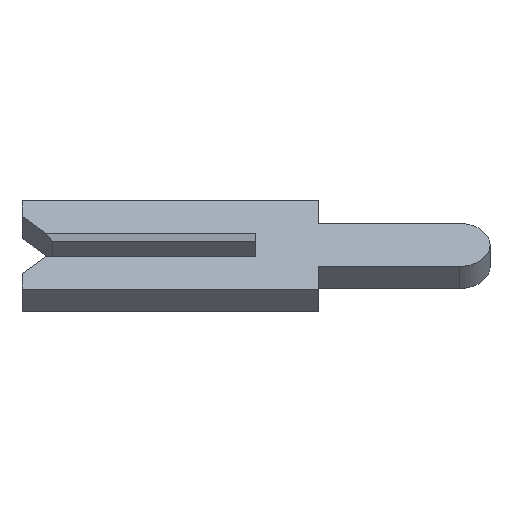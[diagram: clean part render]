
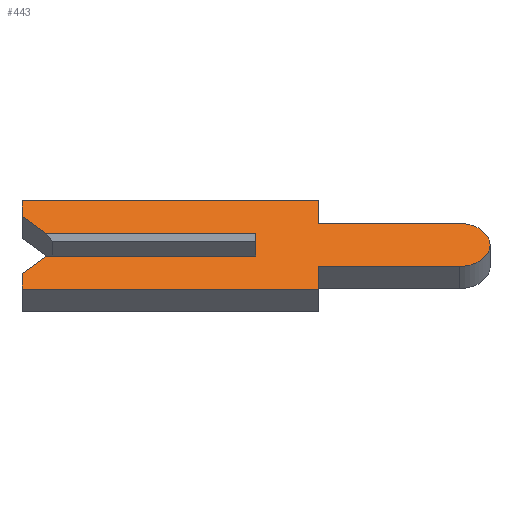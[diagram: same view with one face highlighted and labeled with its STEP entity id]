
A CAD part, left-side view. The second image highlights one B-rep face of the part: STEP entity #443.
In plain terms, the highlighted face is planar.
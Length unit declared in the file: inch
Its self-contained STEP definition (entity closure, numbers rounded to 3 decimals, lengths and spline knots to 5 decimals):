
#8 = CARTESIAN_POINT ( 'NONE',  ( -0.01, -0.1305, -0.0195 ) ) ;
#10 = EDGE_CURVE ( 'NONE', #506, #713, #448, .T. ) ;
#23 = ORIENTED_EDGE ( 'NONE', *, *, #317, .F. ) ;
#28 = EDGE_CURVE ( 'NONE', #657, #783, #858, .T. ) ;
#30 = ORIENTED_EDGE ( 'NONE', *, *, #425, .F. ) ;
#32 = ORIENTED_EDGE ( 'NONE', *, *, #181, .F. ) ;
#33 = DIRECTION ( 'NONE',  ( 0., 0.707, 0.707 ) ) ;
#43 = CARTESIAN_POINT ( 'NONE',  ( -0.01, 0., 0.0065 ) ) ;
#47 = VECTOR ( 'NONE', #300, 39.37008 ) ;
#60 = DIRECTION ( 'NONE',  ( 0., -1., 0. ) ) ;
#61 = VERTEX_POINT ( 'NONE', #837 ) ;
#64 = VERTEX_POINT ( 'NONE', #644 ) ;
#73 = DIRECTION ( 'NONE',  ( 0., 0., 1. ) ) ;
#74 = VERTEX_POINT ( 'NONE', #827 ) ;
#80 = CARTESIAN_POINT ( 'NONE',  ( -0.01, 0.15, -0.04 ) ) ;
#82 = EDGE_CURVE ( 'NONE', #295, #551, #475, .T. ) ;
#84 = CARTESIAN_POINT ( 'NONE',  ( -0.01, 0.15, 0.04 ) ) ;
#87 = EDGE_CURVE ( 'NONE', #61, #506, #397, .T. ) ;
#103 = VECTOR ( 'NONE', #861, 39.37008 ) ;
#104 = DIRECTION ( 'NONE',  ( 0., -1., 0. ) ) ;
#112 = EDGE_CURVE ( 'NONE', #632, #61, #745, .T. ) ;
#124 = VECTOR ( 'NONE', #339, 39.37008 ) ;
#135 = DIRECTION ( 'NONE',  ( 0., 0., 1. ) ) ;
#136 = VERTEX_POINT ( 'NONE', #718 ) ;
#140 = CARTESIAN_POINT ( 'NONE',  ( -0.01, -0.04, -0.0195 ) ) ;
#150 = VECTOR ( 'NONE', #581, 39.37008 ) ;
#155 = CARTESIAN_POINT ( 'NONE',  ( -0.01, 0., -0.01 ) ) ;
#162 = CARTESIAN_POINT ( 'NONE',  ( -0.01, 0., 0.01 ) ) ;
#175 = ORIENTED_EDGE ( 'NONE', *, *, #10, .F. ) ;
#181 = EDGE_CURVE ( 'NONE', #136, #295, #421, .T. ) ;
#184 = CARTESIAN_POINT ( 'NONE',  ( -0.01, -0.04, -0.04 ) ) ;
#187 = EDGE_CURVE ( 'NONE', #814, #783, #195, .T. ) ;
#195 = LINE ( 'NONE', #855, #483 ) ;
#204 = CARTESIAN_POINT ( 'NONE',  ( -0.01, 0.15, 0.026 ) ) ;
#211 = LINE ( 'NONE', #501, #492 ) ;
#222 = CARTESIAN_POINT ( 'NONE',  ( -0.01, -0.1305, 0.0195 ) ) ;
#230 = EDGE_CURVE ( 'NONE', #74, #64, #803, .T. ) ;
#243 = VECTOR ( 'NONE', #324, 39.37008 ) ;
#244 = LINE ( 'NONE', #340, #256 ) ;
#246 = CARTESIAN_POINT ( 'NONE',  ( -0.01, 0.15, -0.04 ) ) ;
#255 = CARTESIAN_POINT ( 'NONE',  ( -0.01, -0.1305, 0. ) ) ;
#256 = VECTOR ( 'NONE', #135, 39.37008 ) ;
#263 = DIRECTION ( 'NONE',  ( 1., 0., 0. ) ) ;
#270 = EDGE_CURVE ( 'NONE', #713, #361, #284, .T. ) ;
#275 = LINE ( 'NONE', #568, #810 ) ;
#284 = CIRCLE ( 'NONE', #518, 0.0195 ) ;
#287 = ORIENTED_EDGE ( 'NONE', *, *, #87, .F. ) ;
#288 = ORIENTED_EDGE ( 'NONE', *, *, #112, .F. ) ;
#290 = VERTEX_POINT ( 'NONE', #204 ) ;
#295 = VERTEX_POINT ( 'NONE', #396 ) ;
#300 = DIRECTION ( 'NONE',  ( 0., 1., 0. ) ) ;
#308 = CARTESIAN_POINT ( 'NONE',  ( -0.01, -0.04, 0.0195 ) ) ;
#317 = EDGE_CURVE ( 'NONE', #361, #136, #559, .T. ) ;
#324 = DIRECTION ( 'NONE',  ( 0., 0., -1. ) ) ;
#335 = ORIENTED_EDGE ( 'NONE', *, *, #719, .F. ) ;
#339 = DIRECTION ( 'NONE',  ( 0., 1., 0. ) ) ;
#340 = CARTESIAN_POINT ( 'NONE',  ( -0.01, 0.15, 0.026 ) ) ;
#359 = EDGE_LOOP ( 'NONE', ( #393, #693, #414, #743, #30, #622, #32, #23, #734, #175, #287, #288, #464, #335 ) ) ;
#361 = VERTEX_POINT ( 'NONE', #8 ) ;
#376 = VECTOR ( 'NONE', #73, 39.37008 ) ;
#393 = ORIENTED_EDGE ( 'NONE', *, *, #187, .T. ) ;
#394 = CARTESIAN_POINT ( 'NONE',  ( -0.01, 0.15, 0.04 ) ) ;
#396 = CARTESIAN_POINT ( 'NONE',  ( -0.01, -0.04, -0.04 ) ) ;
#397 = LINE ( 'NONE', #787, #243 ) ;
#412 = AXIS2_PLACEMENT_3D ( 'NONE', #799, #673, #802 ) ;
#414 = ORIENTED_EDGE ( 'NONE', *, *, #796, .F. ) ;
#421 = LINE ( 'NONE', #184, #829 ) ;
#425 = EDGE_CURVE ( 'NONE', #551, #74, #756, .T. ) ;
#432 = FACE_OUTER_BOUND ( 'NONE', #359, .T. ) ;
#443 = ADVANCED_FACE ( 'NONE', ( #432 ), #468, .F. ) ;
#446 = EDGE_CURVE ( 'NONE', #290, #632, #244, .T. ) ;
#448 = LINE ( 'NONE', #308, #729 ) ;
#461 = VECTOR ( 'NONE', #656, 39.37008 ) ;
#462 = CARTESIAN_POINT ( 'NONE',  ( -0.01, 0.15, -0.026 ) ) ;
#464 = ORIENTED_EDGE ( 'NONE', *, *, #446, .F. ) ;
#468 = PLANE ( 'NONE',  #412 ) ;
#475 = LINE ( 'NONE', #246, #47 ) ;
#483 = VECTOR ( 'NONE', #60, 39.37008 ) ;
#492 = VECTOR ( 'NONE', #750, 39.37008 ) ;
#501 = CARTESIAN_POINT ( 'NONE',  ( -0.01, -0.1305, -0.01 ) ) ;
#506 = VERTEX_POINT ( 'NONE', #807 ) ;
#518 = AXIS2_PLACEMENT_3D ( 'NONE', #255, #263, #669 ) ;
#551 = VERTEX_POINT ( 'NONE', #80 ) ;
#559 = LINE ( 'NONE', #140, #124 ) ;
#568 = CARTESIAN_POINT ( 'NONE',  ( -0.01, 0.1305, 0.0065 ) ) ;
#581 = DIRECTION ( 'NONE',  ( 0., 0., 1. ) ) ;
#584 = DIRECTION ( 'NONE',  ( 0., 0., -1. ) ) ;
#591 = CARTESIAN_POINT ( 'NONE',  ( -0.01, 0.1305, -0.0065 ) ) ;
#622 = ORIENTED_EDGE ( 'NONE', *, *, #82, .F. ) ;
#630 = CARTESIAN_POINT ( 'NONE',  ( -0.01, 0.134, 0.01 ) ) ;
#632 = VERTEX_POINT ( 'NONE', #84 ) ;
#644 = CARTESIAN_POINT ( 'NONE',  ( -0.01, 0.134, -0.01 ) ) ;
#656 = DIRECTION ( 'NONE',  ( 0., -0.707, 0.707 ) ) ;
#657 = VERTEX_POINT ( 'NONE', #155 ) ;
#669 = DIRECTION ( 'NONE',  ( 0., 0., -1. ) ) ;
#673 = DIRECTION ( 'NONE',  ( 1., 0., 0. ) ) ;
#693 = ORIENTED_EDGE ( 'NONE', *, *, #28, .F. ) ;
#713 = VERTEX_POINT ( 'NONE', #222 ) ;
#718 = CARTESIAN_POINT ( 'NONE',  ( -0.01, -0.04, -0.0195 ) ) ;
#719 = EDGE_CURVE ( 'NONE', #814, #290, #275, .T. ) ;
#729 = VECTOR ( 'NONE', #104, 39.37008 ) ;
#734 = ORIENTED_EDGE ( 'NONE', *, *, #270, .F. ) ;
#743 = ORIENTED_EDGE ( 'NONE', *, *, #230, .F. ) ;
#745 = LINE ( 'NONE', #394, #103 ) ;
#750 = DIRECTION ( 'NONE',  ( 0., -1., 0. ) ) ;
#756 = LINE ( 'NONE', #462, #376 ) ;
#783 = VERTEX_POINT ( 'NONE', #162 ) ;
#787 = CARTESIAN_POINT ( 'NONE',  ( -0.01, -0.04, 0.04 ) ) ;
#796 = EDGE_CURVE ( 'NONE', #64, #657, #211, .T. ) ;
#799 = CARTESIAN_POINT ( 'NONE',  ( -0.01, -0.1305, 0. ) ) ;
#802 = DIRECTION ( 'NONE',  ( 0., 0., -1. ) ) ;
#803 = LINE ( 'NONE', #591, #461 ) ;
#807 = CARTESIAN_POINT ( 'NONE',  ( -0.01, -0.04, 0.0195 ) ) ;
#810 = VECTOR ( 'NONE', #33, 39.37008 ) ;
#814 = VERTEX_POINT ( 'NONE', #630 ) ;
#827 = CARTESIAN_POINT ( 'NONE',  ( -0.01, 0.15, -0.026 ) ) ;
#829 = VECTOR ( 'NONE', #584, 39.37008 ) ;
#837 = CARTESIAN_POINT ( 'NONE',  ( -0.01, -0.04, 0.04 ) ) ;
#855 = CARTESIAN_POINT ( 'NONE',  ( -0.01, 0.15, 0.01 ) ) ;
#858 = LINE ( 'NONE', #43, #150 ) ;
#861 = DIRECTION ( 'NONE',  ( 0., -1., 0. ) ) ;
